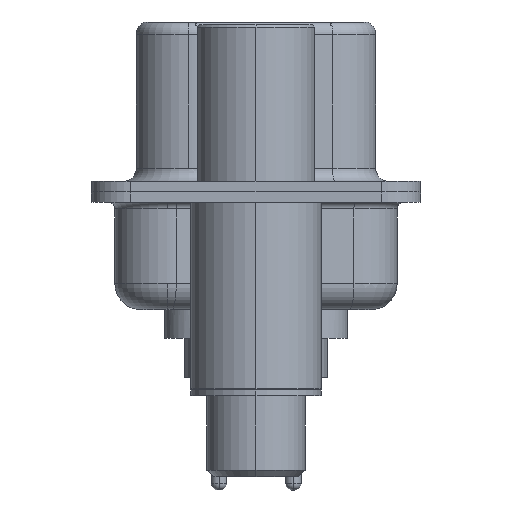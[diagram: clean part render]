
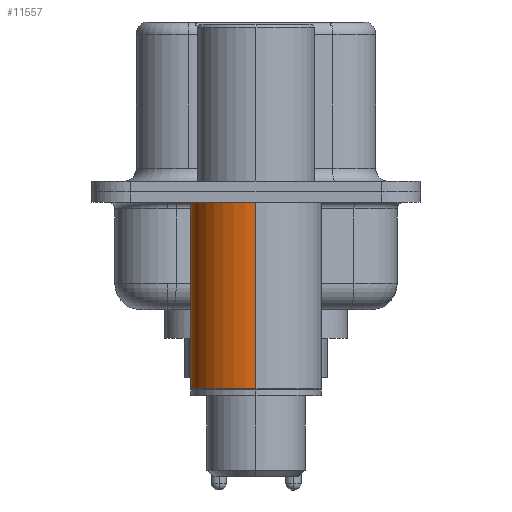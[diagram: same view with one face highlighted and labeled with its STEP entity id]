
A CAD part, left-side view. The second image highlights one B-rep face of the part: STEP entity #11557.
In plain terms, the highlighted cylindrical face has radius 2.5 mm (diameter 5 mm), a partial arc.
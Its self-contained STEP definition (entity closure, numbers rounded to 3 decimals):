
#949 = CARTESIAN_POINT ( 'NONE',  ( 0., 0., -0.4 ) ) ;
#1709 = CARTESIAN_POINT ( 'NONE',  ( -2.5, 0., 0.581 ) ) ;
#1712 = DIRECTION ( 'NONE',  ( 1., 0., 0. ) ) ;
#2204 = LINE ( 'NONE', #10996, #6600 ) ;
#2595 = EDGE_LOOP ( 'NONE', ( #10889, #8144, #16499, #4987 ) ) ;
#2791 = DIRECTION ( 'NONE',  ( 1., 0., 0. ) ) ;
#4987 = ORIENTED_EDGE ( 'NONE', *, *, #20459, .F. ) ;
#5267 = CARTESIAN_POINT ( 'NONE',  ( -2.5, 0., -7.525 ) ) ;
#6600 = VECTOR ( 'NONE', #9089, 1000. ) ;
#7427 = VECTOR ( 'NONE', #14829, 1000. ) ;
#7975 = VERTEX_POINT ( 'NONE', #5267 ) ;
#8144 = ORIENTED_EDGE ( 'NONE', *, *, #21773, .T. ) ;
#8293 = CIRCLE ( 'NONE', #14020, 2.5 ) ;
#8639 = CARTESIAN_POINT ( 'NONE',  ( 0., 0., -7.525 ) ) ;
#8700 = VERTEX_POINT ( 'NONE', #12138 ) ;
#9089 = DIRECTION ( 'NONE',  ( 0., 0., 1. ) ) ;
#10551 = DIRECTION ( 'NONE',  ( 1., 0., 0. ) ) ;
#10679 = CYLINDRICAL_SURFACE ( 'NONE', #22353, 2.5 ) ;
#10889 = ORIENTED_EDGE ( 'NONE', *, *, #12504, .T. ) ;
#10996 = CARTESIAN_POINT ( 'NONE',  ( 2.5, 0., 0.581 ) ) ;
#11107 = DIRECTION ( 'NONE',  ( 0., 0., 1. ) ) ;
#11557 = ADVANCED_FACE ( 'NONE', ( #20771 ), #10679, .T. ) ;
#12138 = CARTESIAN_POINT ( 'NONE',  ( -2.5, 0., -0.4 ) ) ;
#12172 = CARTESIAN_POINT ( 'NONE',  ( 2.5, 0., -7.525 ) ) ;
#12504 = EDGE_CURVE ( 'NONE', #24034, #7975, #8293, .T. ) ;
#12975 = CARTESIAN_POINT ( 'NONE',  ( 0., 0., 0.581 ) ) ;
#13271 = VERTEX_POINT ( 'NONE', #20052 ) ;
#14020 = AXIS2_PLACEMENT_3D ( 'NONE', #8639, #21930, #10551 ) ;
#14054 = DIRECTION ( 'NONE',  ( 0., 0., 1. ) ) ;
#14333 = CIRCLE ( 'NONE', #17873, 2.5 ) ;
#14829 = DIRECTION ( 'NONE',  ( 0., 0., 1. ) ) ;
#15058 = EDGE_CURVE ( 'NONE', #13271, #8700, #14333, .T. ) ;
#16259 = LINE ( 'NONE', #1709, #7427 ) ;
#16499 = ORIENTED_EDGE ( 'NONE', *, *, #15058, .F. ) ;
#17873 = AXIS2_PLACEMENT_3D ( 'NONE', #949, #14054, #2791 ) ;
#20052 = CARTESIAN_POINT ( 'NONE',  ( 2.5, 0., -0.4 ) ) ;
#20459 = EDGE_CURVE ( 'NONE', #24034, #13271, #2204, .T. ) ;
#20771 = FACE_OUTER_BOUND ( 'NONE', #2595, .T. ) ;
#21773 = EDGE_CURVE ( 'NONE', #7975, #8700, #16259, .T. ) ;
#21930 = DIRECTION ( 'NONE',  ( 0., 0., 1. ) ) ;
#22353 = AXIS2_PLACEMENT_3D ( 'NONE', #12975, #11107, #1712 ) ;
#24034 = VERTEX_POINT ( 'NONE', #12172 ) ;
